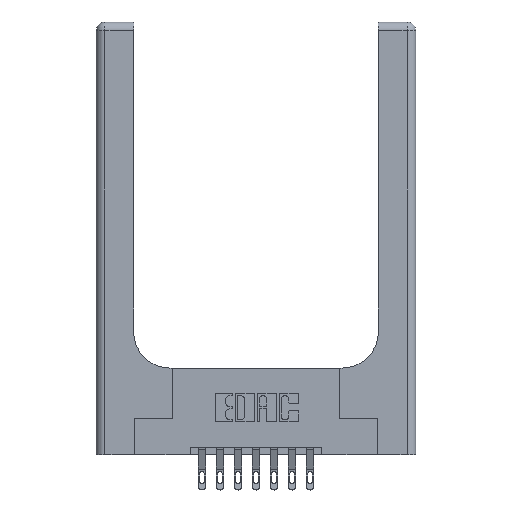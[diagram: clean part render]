
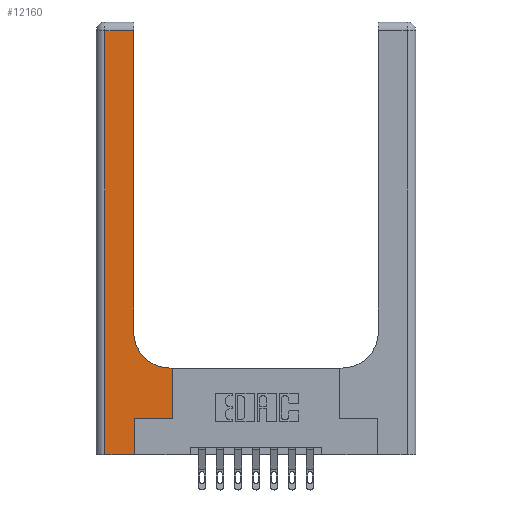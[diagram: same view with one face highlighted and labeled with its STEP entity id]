
A CAD part, top view. The second image highlights one B-rep face of the part: STEP entity #12160.
In plain terms, the highlighted planar face has unit normal (0, 0, 1).
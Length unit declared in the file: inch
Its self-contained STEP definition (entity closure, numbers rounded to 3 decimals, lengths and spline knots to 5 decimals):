
#354 = VECTOR ( 'NONE', #6259, 39.37008 ) ;
#535 = EDGE_CURVE ( 'NONE', #4377, #9886, #12036, .T. ) ;
#720 = ORIENTED_EDGE ( 'NONE', *, *, #14214, .T. ) ;
#919 = CARTESIAN_POINT ( 'NONE',  ( 0.26, 0.85, 0.37 ) ) ;
#949 = DIRECTION ( 'NONE',  ( 0., 0., -1. ) ) ;
#1103 = CARTESIAN_POINT ( 'NONE',  ( 0.265, 0.25, 0.37 ) ) ;
#1172 = DIRECTION ( 'NONE',  ( 0., -1., 0. ) ) ;
#1252 = VECTOR ( 'NONE', #6628, 39.37008 ) ;
#1307 = VECTOR ( 'NONE', #1172, 39.37008 ) ;
#1732 = ORIENTED_EDGE ( 'NONE', *, *, #535, .T. ) ;
#1749 = CARTESIAN_POINT ( 'NONE',  ( 0.26, 2.94, 0.37 ) ) ;
#1778 = ORIENTED_EDGE ( 'NONE', *, *, #6191, .T. ) ;
#1931 = LINE ( 'NONE', #13565, #1252 ) ;
#1946 = VECTOR ( 'NONE', #7029, 39.37008 ) ;
#2041 = ORIENTED_EDGE ( 'NONE', *, *, #8836, .T. ) ;
#2125 = ORIENTED_EDGE ( 'NONE', *, *, #7499, .T. ) ;
#2262 = LINE ( 'NONE', #12957, #1946 ) ;
#2418 = ORIENTED_EDGE ( 'NONE', *, *, #14712, .T. ) ;
#2617 = ORIENTED_EDGE ( 'NONE', *, *, #7037, .T. ) ;
#2838 = EDGE_CURVE ( 'NONE', #15212, #11158, #2262, .T. ) ;
#3157 = CARTESIAN_POINT ( 'NONE',  ( 0., 3., 0.37 ) ) ;
#3304 = DIRECTION ( 'NONE',  ( -1., 0., 0. ) ) ;
#3326 = DIRECTION ( 'NONE',  ( 0., 1., 0. ) ) ;
#3384 = DIRECTION ( 'NONE',  ( -1., 0., 0. ) ) ;
#3771 = CARTESIAN_POINT ( 'NONE',  ( 0.528, 0.25, 0.37 ) ) ;
#4175 = VECTOR ( 'NONE', #3326, 39.37008 ) ;
#4377 = VERTEX_POINT ( 'NONE', #1103 ) ;
#4430 = DIRECTION ( 'NONE',  ( 1., 0., 0. ) ) ;
#4689 = VERTEX_POINT ( 'NONE', #14470 ) ;
#6123 = CARTESIAN_POINT ( 'NONE',  ( 0.06, 3., 0.37 ) ) ;
#6191 = EDGE_CURVE ( 'NONE', #4689, #7640, #9302, .T. ) ;
#6259 = DIRECTION ( 'NONE',  ( 1., 0., 0. ) ) ;
#6628 = DIRECTION ( 'NONE',  ( 0., 1., 0. ) ) ;
#6697 = PLANE ( 'NONE',  #10129 ) ;
#6814 = LINE ( 'NONE', #10342, #15182 ) ;
#6821 = CARTESIAN_POINT ( 'NONE',  ( 0.51, 0.6, 0.37 ) ) ;
#6825 = CARTESIAN_POINT ( 'NONE',  ( 0.51, 0.85, 0.37 ) ) ;
#7029 = DIRECTION ( 'NONE',  ( -1., 0., 0. ) ) ;
#7037 = EDGE_CURVE ( 'NONE', #13138, #15212, #6814, .T. ) ;
#7263 = LINE ( 'NONE', #6123, #1307 ) ;
#7474 = VERTEX_POINT ( 'NONE', #10169 ) ;
#7499 = EDGE_CURVE ( 'NONE', #14010, #4377, #9090, .T. ) ;
#7640 = VERTEX_POINT ( 'NONE', #6821 ) ;
#7871 = ORIENTED_EDGE ( 'NONE', *, *, #2838, .T. ) ;
#8836 = EDGE_CURVE ( 'NONE', #7640, #13138, #14270, .T. ) ;
#9090 = LINE ( 'NONE', #11357, #4175 ) ;
#9130 = EDGE_CURVE ( 'NONE', #7474, #14010, #9657, .T. ) ;
#9146 = FACE_OUTER_BOUND ( 'NONE', #13349, .T. ) ;
#9227 = DIRECTION ( 'NONE',  ( 0., 0., -1. ) ) ;
#9302 = LINE ( 'NONE', #10023, #14678 ) ;
#9558 = CARTESIAN_POINT ( 'NONE',  ( 0.265, 0.25, 0.37 ) ) ;
#9657 = LINE ( 'NONE', #14358, #11627 ) ;
#9886 = VERTEX_POINT ( 'NONE', #3771 ) ;
#10023 = CARTESIAN_POINT ( 'NONE',  ( 0.26, 0.6, 0.37 ) ) ;
#10129 = AXIS2_PLACEMENT_3D ( 'NONE', #3157, #9227, #3384 ) ;
#10169 = CARTESIAN_POINT ( 'NONE',  ( 0.06, 0., 0.37 ) ) ;
#10342 = CARTESIAN_POINT ( 'NONE',  ( 0.26, 3., 0.37 ) ) ;
#10572 = AXIS2_PLACEMENT_3D ( 'NONE', #6825, #949, #11386 ) ;
#11063 = CARTESIAN_POINT ( 'NONE',  ( 0.265, 0., 0.37 ) ) ;
#11158 = VERTEX_POINT ( 'NONE', #13248 ) ;
#11357 = CARTESIAN_POINT ( 'NONE',  ( 0.265, 0., 0.37 ) ) ;
#11386 = DIRECTION ( 'NONE',  ( 1., 0., 0. ) ) ;
#11627 = VECTOR ( 'NONE', #4430, 39.37008 ) ;
#12036 = LINE ( 'NONE', #9558, #354 ) ;
#12160 = ADVANCED_FACE ( 'NONE', ( #9146 ), #6697, .F. ) ;
#12516 = DIRECTION ( 'NONE',  ( 0., 1., 0. ) ) ;
#12957 = CARTESIAN_POINT ( 'NONE',  ( 0., 2.94, 0.37 ) ) ;
#13138 = VERTEX_POINT ( 'NONE', #919 ) ;
#13248 = CARTESIAN_POINT ( 'NONE',  ( 0.06, 2.94, 0.37 ) ) ;
#13349 = EDGE_LOOP ( 'NONE', ( #2617, #7871, #720, #14449, #2125, #1732, #2418, #1778, #2041 ) ) ;
#13565 = CARTESIAN_POINT ( 'NONE',  ( 0.528, 0.25, 0.37 ) ) ;
#14010 = VERTEX_POINT ( 'NONE', #11063 ) ;
#14214 = EDGE_CURVE ( 'NONE', #11158, #7474, #7263, .T. ) ;
#14270 = CIRCLE ( 'NONE', #10572, 0.25 ) ;
#14358 = CARTESIAN_POINT ( 'NONE',  ( 0., 0., 0.37 ) ) ;
#14449 = ORIENTED_EDGE ( 'NONE', *, *, #9130, .T. ) ;
#14470 = CARTESIAN_POINT ( 'NONE',  ( 0.528, 0.6, 0.37 ) ) ;
#14678 = VECTOR ( 'NONE', #3304, 39.37008 ) ;
#14712 = EDGE_CURVE ( 'NONE', #9886, #4689, #1931, .T. ) ;
#15182 = VECTOR ( 'NONE', #12516, 39.37008 ) ;
#15212 = VERTEX_POINT ( 'NONE', #1749 ) ;
